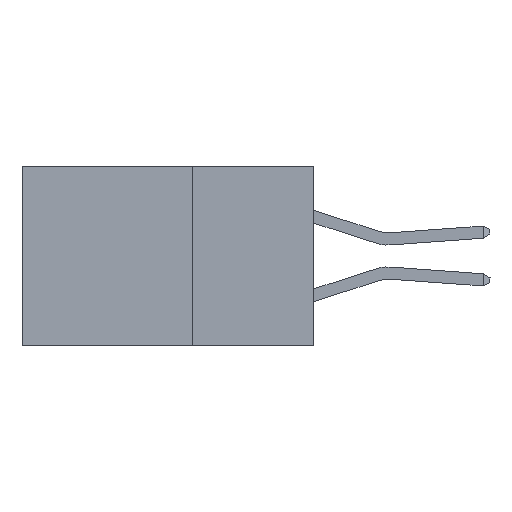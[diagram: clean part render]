
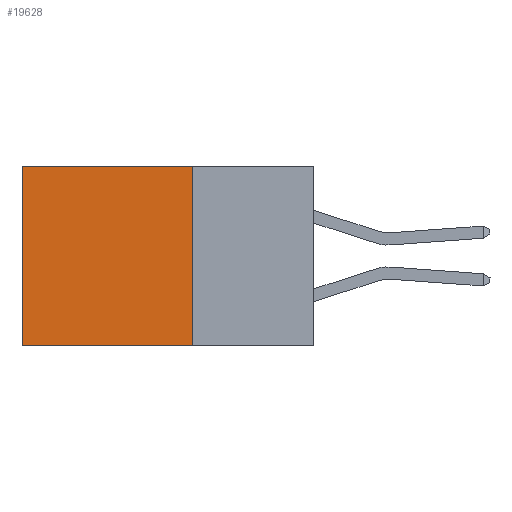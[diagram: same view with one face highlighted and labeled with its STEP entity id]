
A CAD part, left-side view. The second image highlights one B-rep face of the part: STEP entity #19628.
In plain terms, the highlighted planar face has unit normal (-1, 0, 0).
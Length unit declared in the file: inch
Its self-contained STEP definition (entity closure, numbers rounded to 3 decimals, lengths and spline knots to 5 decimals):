
#3302 = CARTESIAN_POINT ( 'NONE',  ( 0.2875, 0.25, -0.37 ) ) ;
#3460 = ORIENTED_EDGE ( 'NONE', *, *, #26606, .T. ) ;
#3869 = PLANE ( 'NONE',  #7272 ) ;
#5206 = FACE_OUTER_BOUND ( 'NONE', #21434, .T. ) ;
#5257 = CARTESIAN_POINT ( 'NONE',  ( 0.2875, 0.6, 0. ) ) ;
#5418 = EDGE_CURVE ( 'NONE', #18426, #24864, #24720, .T. ) ;
#5781 = EDGE_CURVE ( 'NONE', #24864, #14103, #25694, .T. ) ;
#7272 = AXIS2_PLACEMENT_3D ( 'NONE', #24901, #12495, #14348 ) ;
#7351 = EDGE_CURVE ( 'NONE', #9382, #14103, #11142, .T. ) ;
#7602 = CARTESIAN_POINT ( 'NONE',  ( 0.2875, 0.25, 0. ) ) ;
#7914 = CARTESIAN_POINT ( 'NONE',  ( 0.2875, 0.6, -0.37 ) ) ;
#8227 = VECTOR ( 'NONE', #22116, 39.37008 ) ;
#8388 = CARTESIAN_POINT ( 'NONE',  ( 0.2875, 0.25, 0. ) ) ;
#8941 = ORIENTED_EDGE ( 'NONE', *, *, #7351, .T. ) ;
#9369 = DIRECTION ( 'NONE',  ( 0., 1., 0. ) ) ;
#9382 = VERTEX_POINT ( 'NONE', #26905 ) ;
#11142 = LINE ( 'NONE', #5257, #8227 ) ;
#11523 = DIRECTION ( 'NONE',  ( 0., 1., 0. ) ) ;
#11572 = ORIENTED_EDGE ( 'NONE', *, *, #5418, .F. ) ;
#12495 = DIRECTION ( 'NONE',  ( 1., 0., 0. ) ) ;
#12740 = CARTESIAN_POINT ( 'NONE',  ( 0.2875, 0.25, 0. ) ) ;
#13095 = LINE ( 'NONE', #7602, #14138 ) ;
#14103 = VERTEX_POINT ( 'NONE', #7914 ) ;
#14138 = VECTOR ( 'NONE', #11523, 39.37008 ) ;
#14348 = DIRECTION ( 'NONE',  ( 0., 0., -1. ) ) ;
#17831 = ORIENTED_EDGE ( 'NONE', *, *, #5781, .F. ) ;
#18426 = VERTEX_POINT ( 'NONE', #12740 ) ;
#19628 = ADVANCED_FACE ( 'NONE', ( #5206 ), #3869, .F. ) ;
#21434 = EDGE_LOOP ( 'NONE', ( #8941, #17831, #11572, #3460 ) ) ;
#22022 = CARTESIAN_POINT ( 'NONE',  ( 0.2875, 0.25, -0.37 ) ) ;
#22116 = DIRECTION ( 'NONE',  ( 0., 0., -1. ) ) ;
#22122 = VECTOR ( 'NONE', #9369, 39.37008 ) ;
#22463 = VECTOR ( 'NONE', #22901, 39.37008 ) ;
#22901 = DIRECTION ( 'NONE',  ( 0., 0., -1. ) ) ;
#24720 = LINE ( 'NONE', #8388, #22463 ) ;
#24864 = VERTEX_POINT ( 'NONE', #22022 ) ;
#24901 = CARTESIAN_POINT ( 'NONE',  ( 0.2875, 0.25, 0. ) ) ;
#25694 = LINE ( 'NONE', #3302, #22122 ) ;
#26606 = EDGE_CURVE ( 'NONE', #18426, #9382, #13095, .T. ) ;
#26905 = CARTESIAN_POINT ( 'NONE',  ( 0.2875, 0.6, 0. ) ) ;
